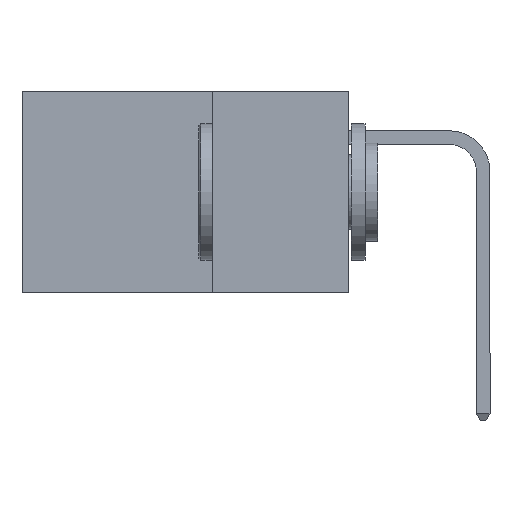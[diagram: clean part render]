
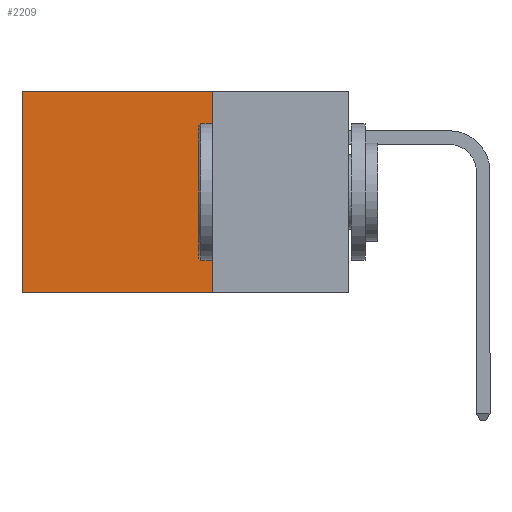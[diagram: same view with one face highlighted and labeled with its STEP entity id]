
A CAD part, left-side view. The second image highlights one B-rep face of the part: STEP entity #2209.
In plain terms, the highlighted planar face has unit normal (-1, 0, 0).
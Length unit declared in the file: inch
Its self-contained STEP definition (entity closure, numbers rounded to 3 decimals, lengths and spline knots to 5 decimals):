
#217 = VERTEX_POINT ( 'NONE', #8402 ) ;
#257 = VERTEX_POINT ( 'NONE', #7550 ) ;
#870 = EDGE_CURVE ( 'NONE', #1565, #3675, #8308, .T. ) ;
#1565 = VERTEX_POINT ( 'NONE', #9133 ) ;
#2209 = ADVANCED_FACE ( 'NONE', ( #8601 ), #5965, .F. ) ;
#2229 = VECTOR ( 'NONE', #6139, 39.37008 ) ;
#2455 = CARTESIAN_POINT ( 'NONE',  ( 0.2875, 0.6, 0. ) ) ;
#2468 = DIRECTION ( 'NONE',  ( 0., 0., -1. ) ) ;
#2603 = VECTOR ( 'NONE', #3361, 39.37008 ) ;
#2623 = DIRECTION ( 'NONE',  ( 0., 1., 0. ) ) ;
#2656 = ORIENTED_EDGE ( 'NONE', *, *, #870, .T. ) ;
#2706 = ORIENTED_EDGE ( 'NONE', *, *, #9420, .F. ) ;
#2715 = ORIENTED_EDGE ( 'NONE', *, *, #7110, .F. ) ;
#2762 = ORIENTED_EDGE ( 'NONE', *, *, #3504, .T. ) ;
#2884 = LINE ( 'NONE', #7981, #2603 ) ;
#3361 = DIRECTION ( 'NONE',  ( 0., 0., -1. ) ) ;
#3504 = EDGE_CURVE ( 'NONE', #257, #1565, #6592, .T. ) ;
#3675 = VERTEX_POINT ( 'NONE', #5334 ) ;
#5334 = CARTESIAN_POINT ( 'NONE',  ( 0.2875, 0.6, -0.37 ) ) ;
#5443 = DIRECTION ( 'NONE',  ( 0., 0., -1. ) ) ;
#5620 = DIRECTION ( 'NONE',  ( 1., 0., 0. ) ) ;
#5687 = CARTESIAN_POINT ( 'NONE',  ( 0.2875, 0.25, 0. ) ) ;
#5965 = PLANE ( 'NONE',  #8657 ) ;
#6139 = DIRECTION ( 'NONE',  ( 0., 1., 0. ) ) ;
#6152 = CARTESIAN_POINT ( 'NONE',  ( 0.2875, 0.25, 0. ) ) ;
#6185 = VECTOR ( 'NONE', #2468, 39.37008 ) ;
#6592 = LINE ( 'NONE', #6152, #2229 ) ;
#6979 = LINE ( 'NONE', #7409, #8631 ) ;
#7110 = EDGE_CURVE ( 'NONE', #257, #217, #2884, .T. ) ;
#7409 = CARTESIAN_POINT ( 'NONE',  ( 0.2875, 0.25, -0.37 ) ) ;
#7550 = CARTESIAN_POINT ( 'NONE',  ( 0.2875, 0.25, 0. ) ) ;
#7981 = CARTESIAN_POINT ( 'NONE',  ( 0.2875, 0.25, 0. ) ) ;
#8308 = LINE ( 'NONE', #2455, #6185 ) ;
#8402 = CARTESIAN_POINT ( 'NONE',  ( 0.2875, 0.25, -0.37 ) ) ;
#8601 = FACE_OUTER_BOUND ( 'NONE', #9916, .T. ) ;
#8631 = VECTOR ( 'NONE', #2623, 39.37008 ) ;
#8657 = AXIS2_PLACEMENT_3D ( 'NONE', #5687, #5620, #5443 ) ;
#9133 = CARTESIAN_POINT ( 'NONE',  ( 0.2875, 0.6, 0. ) ) ;
#9420 = EDGE_CURVE ( 'NONE', #217, #3675, #6979, .T. ) ;
#9916 = EDGE_LOOP ( 'NONE', ( #2656, #2706, #2715, #2762 ) ) ;
